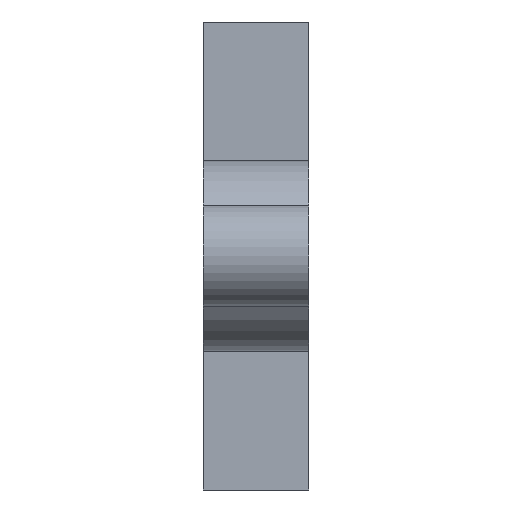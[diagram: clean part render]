
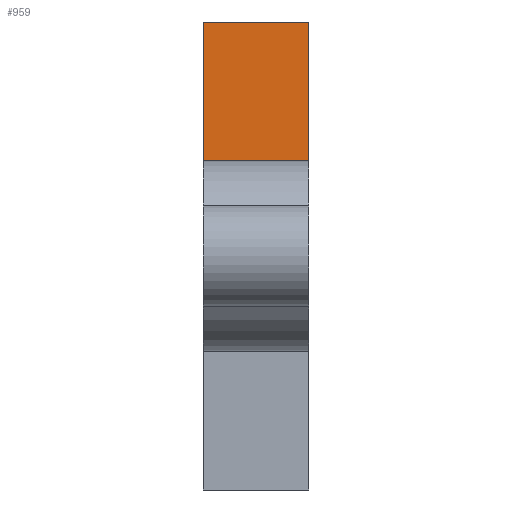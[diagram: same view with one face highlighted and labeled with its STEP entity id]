
A CAD part, front view. The second image highlights one B-rep face of the part: STEP entity #959.
In plain terms, the highlighted planar face has unit normal (0, -1, 0).
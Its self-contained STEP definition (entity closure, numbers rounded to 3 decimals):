
#5 = ORIENTED_EDGE ( 'NONE', *, *, #461, .T. ) ;
#30 = VERTEX_POINT ( 'NONE', #1002 ) ;
#52 = CARTESIAN_POINT ( 'NONE',  ( 0.33, -2.515, 1.461 ) ) ;
#96 = DIRECTION ( 'NONE',  ( 0., 0., 1. ) ) ;
#137 = LINE ( 'NONE', #52, #199 ) ;
#199 = VECTOR ( 'NONE', #743, 1000. ) ;
#216 = ORIENTED_EDGE ( 'NONE', *, *, #936, .F. ) ;
#219 = AXIS2_PLACEMENT_3D ( 'NONE', #274, #362, #96 ) ;
#225 = DIRECTION ( 'NONE',  ( 0., 0., -1. ) ) ;
#233 = VECTOR ( 'NONE', #769, 1000. ) ;
#251 = CARTESIAN_POINT ( 'NONE',  ( 0.33, -2.515, 0.597 ) ) ;
#274 = CARTESIAN_POINT ( 'NONE',  ( 0.33, -2.515, 1.461 ) ) ;
#277 = PLANE ( 'NONE',  #219 ) ;
#362 = DIRECTION ( 'NONE',  ( 0., 1., 0. ) ) ;
#426 = LINE ( 'NONE', #938, #1016 ) ;
#461 = EDGE_CURVE ( 'NONE', #1043, #685, #719, .T. ) ;
#545 = DIRECTION ( 'NONE',  ( 0., 0., -1. ) ) ;
#600 = FACE_OUTER_BOUND ( 'NONE', #986, .T. ) ;
#614 = ORIENTED_EDGE ( 'NONE', *, *, #865, .F. ) ;
#685 = VERTEX_POINT ( 'NONE', #1058 ) ;
#701 = CARTESIAN_POINT ( 'NONE',  ( -0.33, -2.515, 1.461 ) ) ;
#719 = LINE ( 'NONE', #964, #995 ) ;
#743 = DIRECTION ( 'NONE',  ( -1., 0., 0. ) ) ;
#760 = EDGE_CURVE ( 'NONE', #973, #1043, #137, .T. ) ;
#769 = DIRECTION ( 'NONE',  ( -1., 0., 0. ) ) ;
#781 = ORIENTED_EDGE ( 'NONE', *, *, #760, .T. ) ;
#865 = EDGE_CURVE ( 'NONE', #30, #685, #1055, .T. ) ;
#936 = EDGE_CURVE ( 'NONE', #973, #30, #426, .T. ) ;
#938 = CARTESIAN_POINT ( 'NONE',  ( 0.33, -2.515, 1.461 ) ) ;
#946 = CARTESIAN_POINT ( 'NONE',  ( 0.33, -2.515, 1.461 ) ) ;
#959 = ADVANCED_FACE ( 'NONE', ( #600 ), #277, .F. ) ;
#964 = CARTESIAN_POINT ( 'NONE',  ( -0.33, -2.515, 1.461 ) ) ;
#973 = VERTEX_POINT ( 'NONE', #946 ) ;
#986 = EDGE_LOOP ( 'NONE', ( #5, #614, #216, #781 ) ) ;
#995 = VECTOR ( 'NONE', #225, 1000. ) ;
#1002 = CARTESIAN_POINT ( 'NONE',  ( 0.33, -2.515, 0.597 ) ) ;
#1016 = VECTOR ( 'NONE', #545, 1000. ) ;
#1043 = VERTEX_POINT ( 'NONE', #701 ) ;
#1055 = LINE ( 'NONE', #251, #233 ) ;
#1058 = CARTESIAN_POINT ( 'NONE',  ( -0.33, -2.515, 0.597 ) ) ;
